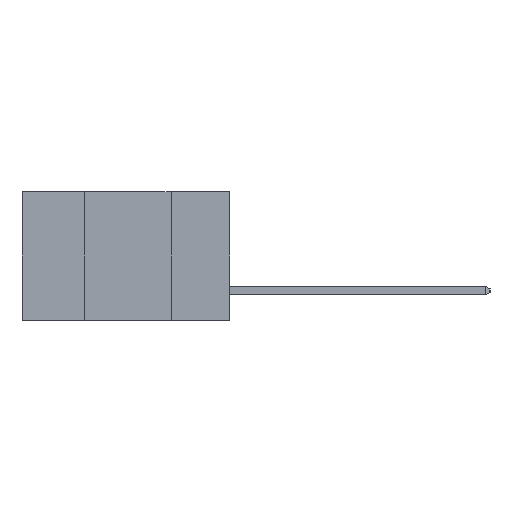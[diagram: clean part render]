
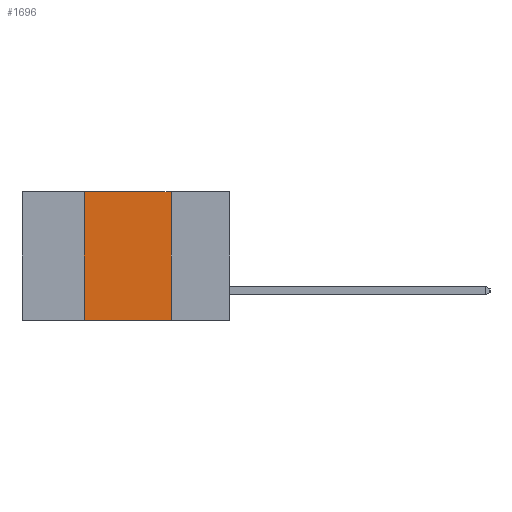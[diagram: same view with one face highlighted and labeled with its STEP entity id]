
A CAD part, left-side view. The second image highlights one B-rep face of the part: STEP entity #1696.
In plain terms, the highlighted planar face has unit normal (-1, 0, 0).
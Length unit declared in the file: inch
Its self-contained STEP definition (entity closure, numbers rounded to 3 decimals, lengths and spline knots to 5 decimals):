
#114 = PLANE ( 'NONE',  #1534 ) ;
#769 = CARTESIAN_POINT ( 'NONE',  ( 0., 0.42, -0.37 ) ) ;
#786 = CARTESIAN_POINT ( 'NONE',  ( 0., 0.42, 0. ) ) ;
#788 = DIRECTION ( 'NONE',  ( 1., 0., 0. ) ) ;
#802 = DIRECTION ( 'NONE',  ( 0., 0., 1. ) ) ;
#1443 = LINE ( 'NONE', #8427, #4470 ) ;
#1534 = AXIS2_PLACEMENT_3D ( 'NONE', #5715, #788, #11661 ) ;
#1696 = ADVANCED_FACE ( 'NONE', ( #3713 ), #114, .F. ) ;
#2235 = LINE ( 'NONE', #9204, #10299 ) ;
#2490 = DIRECTION ( 'NONE',  ( 0., -1., 0. ) ) ;
#2706 = VECTOR ( 'NONE', #7241, 39.37008 ) ;
#2754 = EDGE_CURVE ( 'NONE', #4659, #10387, #7286, .T. ) ;
#3604 = EDGE_CURVE ( 'NONE', #10387, #12481, #1443, .T. ) ;
#3713 = FACE_OUTER_BOUND ( 'NONE', #12955, .T. ) ;
#4057 = ORIENTED_EDGE ( 'NONE', *, *, #9104, .T. ) ;
#4382 = CARTESIAN_POINT ( 'NONE',  ( 0., 0.17, -0.37 ) ) ;
#4470 = VECTOR ( 'NONE', #2490, 39.37008 ) ;
#4659 = VERTEX_POINT ( 'NONE', #769 ) ;
#5263 = ORIENTED_EDGE ( 'NONE', *, *, #2754, .F. ) ;
#5341 = ORIENTED_EDGE ( 'NONE', *, *, #3604, .F. ) ;
#5385 = ORIENTED_EDGE ( 'NONE', *, *, #11532, .F. ) ;
#5575 = VERTEX_POINT ( 'NONE', #4382 ) ;
#5715 = CARTESIAN_POINT ( 'NONE',  ( 0., 0.6, 0. ) ) ;
#7241 = DIRECTION ( 'NONE',  ( 0., 0., -1. ) ) ;
#7286 = LINE ( 'NONE', #786, #11821 ) ;
#8117 = CARTESIAN_POINT ( 'NONE',  ( 0., 0.17, 0. ) ) ;
#8427 = CARTESIAN_POINT ( 'NONE',  ( 0., 0.6, 0. ) ) ;
#9104 = EDGE_CURVE ( 'NONE', #4659, #5575, #2235, .T. ) ;
#9163 = CARTESIAN_POINT ( 'NONE',  ( 0., 0.17, 0. ) ) ;
#9204 = CARTESIAN_POINT ( 'NONE',  ( 0., 0.6, -0.37 ) ) ;
#10223 = DIRECTION ( 'NONE',  ( 0., -1., 0. ) ) ;
#10299 = VECTOR ( 'NONE', #10223, 39.37008 ) ;
#10387 = VERTEX_POINT ( 'NONE', #10482 ) ;
#10482 = CARTESIAN_POINT ( 'NONE',  ( 0., 0.42, 0. ) ) ;
#11532 = EDGE_CURVE ( 'NONE', #12481, #5575, #11662, .T. ) ;
#11661 = DIRECTION ( 'NONE',  ( 0., 0., -1. ) ) ;
#11662 = LINE ( 'NONE', #9163, #2706 ) ;
#11821 = VECTOR ( 'NONE', #802, 39.37008 ) ;
#12481 = VERTEX_POINT ( 'NONE', #8117 ) ;
#12955 = EDGE_LOOP ( 'NONE', ( #5385, #5341, #5263, #4057 ) ) ;
